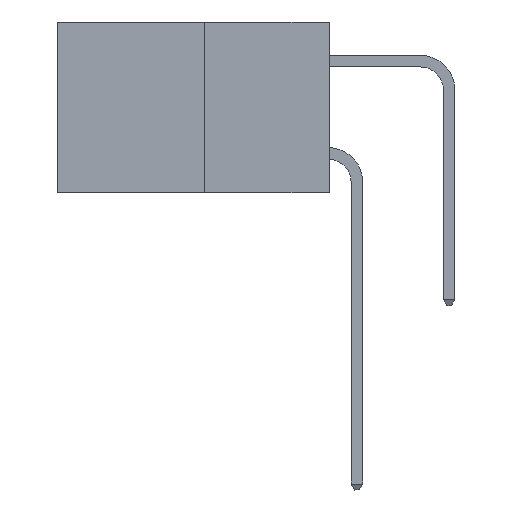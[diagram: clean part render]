
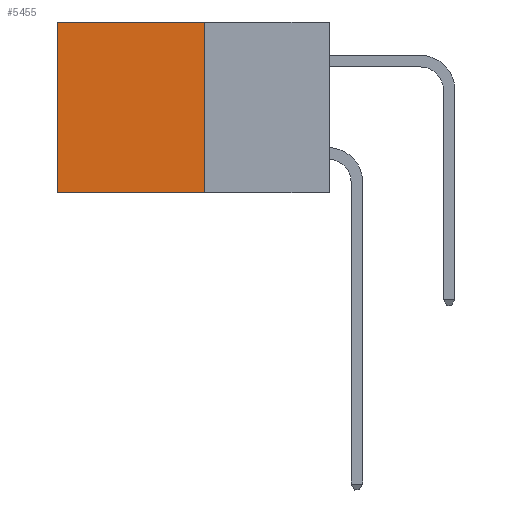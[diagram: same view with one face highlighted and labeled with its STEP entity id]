
A CAD part, left-side view. The second image highlights one B-rep face of the part: STEP entity #5455.
In plain terms, the highlighted planar face has unit normal (-1, 0, 0).
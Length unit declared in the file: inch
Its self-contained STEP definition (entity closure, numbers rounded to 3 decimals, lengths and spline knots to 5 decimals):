
#588 = CARTESIAN_POINT ( 'NONE',  ( 0.277, 0.27, -0.37 ) ) ;
#1217 = VERTEX_POINT ( 'NONE', #31729 ) ;
#1558 = CARTESIAN_POINT ( 'NONE',  ( 0.277, 0.59, -0.37 ) ) ;
#2970 = EDGE_CURVE ( 'NONE', #1217, #7955, #15853, .T. ) ;
#3399 = DIRECTION ( 'NONE',  ( 0., 1., 0. ) ) ;
#3739 = VERTEX_POINT ( 'NONE', #14771 ) ;
#5455 = ADVANCED_FACE ( 'NONE', ( #32032 ), #9667, .F. ) ;
#6038 = CARTESIAN_POINT ( 'NONE',  ( 0.277, 0.27, -0.37 ) ) ;
#7955 = VERTEX_POINT ( 'NONE', #1558 ) ;
#8251 = VECTOR ( 'NONE', #33905, 39.37008 ) ;
#9345 = CARTESIAN_POINT ( 'NONE',  ( 0.277, 0.27, -0.37 ) ) ;
#9667 = PLANE ( 'NONE',  #21593 ) ;
#10028 = DIRECTION ( 'NONE',  ( 0., 0., -1. ) ) ;
#10034 = DIRECTION ( 'NONE',  ( 1., 0., 0. ) ) ;
#11295 = ORIENTED_EDGE ( 'NONE', *, *, #31899, .F. ) ;
#13084 = ORIENTED_EDGE ( 'NONE', *, *, #24689, .F. ) ;
#13836 = DIRECTION ( 'NONE',  ( 0., 1., 0. ) ) ;
#14771 = CARTESIAN_POINT ( 'NONE',  ( 0.277, 0.27, 0. ) ) ;
#15853 = LINE ( 'NONE', #34388, #8251 ) ;
#16990 = VECTOR ( 'NONE', #35337, 39.37008 ) ;
#17844 = VERTEX_POINT ( 'NONE', #6038 ) ;
#20208 = ORIENTED_EDGE ( 'NONE', *, *, #2970, .T. ) ;
#21593 = AXIS2_PLACEMENT_3D ( 'NONE', #9345, #10034, #10028 ) ;
#21761 = LINE ( 'NONE', #588, #28229 ) ;
#22850 = LINE ( 'NONE', #24865, #28395 ) ;
#24689 = EDGE_CURVE ( 'NONE', #3739, #17844, #31524, .T. ) ;
#24865 = CARTESIAN_POINT ( 'NONE',  ( 0.277, 0.27, 0. ) ) ;
#25622 = ORIENTED_EDGE ( 'NONE', *, *, #29772, .T. ) ;
#28229 = VECTOR ( 'NONE', #3399, 39.37008 ) ;
#28395 = VECTOR ( 'NONE', #13836, 39.37008 ) ;
#29772 = EDGE_CURVE ( 'NONE', #3739, #1217, #22850, .T. ) ;
#31043 = EDGE_LOOP ( 'NONE', ( #20208, #11295, #13084, #25622 ) ) ;
#31524 = LINE ( 'NONE', #32601, #16990 ) ;
#31729 = CARTESIAN_POINT ( 'NONE',  ( 0.277, 0.59, 0. ) ) ;
#31899 = EDGE_CURVE ( 'NONE', #17844, #7955, #21761, .T. ) ;
#32032 = FACE_OUTER_BOUND ( 'NONE', #31043, .T. ) ;
#32601 = CARTESIAN_POINT ( 'NONE',  ( 0.277, 0.27, -0.37 ) ) ;
#33905 = DIRECTION ( 'NONE',  ( 0., 0., -1. ) ) ;
#34388 = CARTESIAN_POINT ( 'NONE',  ( 0.277, 0.59, -0.37 ) ) ;
#35337 = DIRECTION ( 'NONE',  ( 0., 0., -1. ) ) ;
